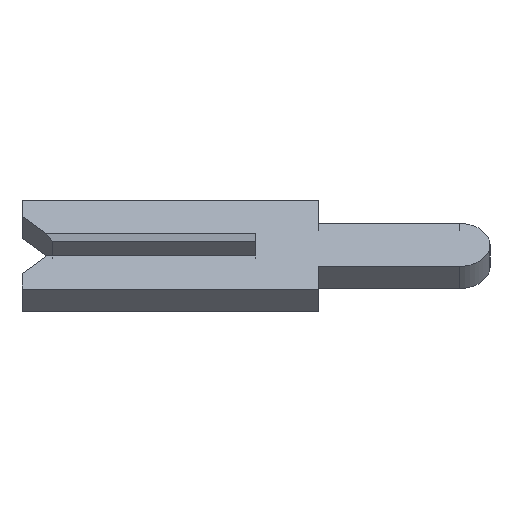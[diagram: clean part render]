
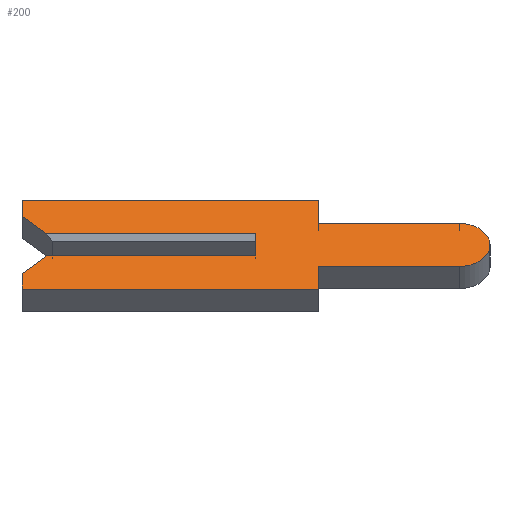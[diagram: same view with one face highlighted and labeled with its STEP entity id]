
A CAD part, left-side view. The second image highlights one B-rep face of the part: STEP entity #200.
In plain terms, the highlighted face is planar.
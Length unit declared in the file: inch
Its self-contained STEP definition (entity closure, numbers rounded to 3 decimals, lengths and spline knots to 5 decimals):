
#16 = LINE ( 'NONE', #425, #167 ) ;
#18 = CARTESIAN_POINT ( 'NONE',  ( -0.01, -0.1305, -0.0195 ) ) ;
#24 = ORIENTED_EDGE ( 'NONE', *, *, #143, .F. ) ;
#27 = PLANE ( 'NONE',  #1065 ) ;
#28 = ORIENTED_EDGE ( 'NONE', *, *, #935, .F. ) ;
#33 = LINE ( 'NONE', #1054, #142 ) ;
#55 = ORIENTED_EDGE ( 'NONE', *, *, #101, .F. ) ;
#59 = VERTEX_POINT ( 'NONE', #343 ) ;
#66 = VERTEX_POINT ( 'NONE', #703 ) ;
#69 = ORIENTED_EDGE ( 'NONE', *, *, #1071, .F. ) ;
#80 = DIRECTION ( 'NONE',  ( 1., 0., 0. ) ) ;
#82 = VECTOR ( 'NONE', #792, 39.37008 ) ;
#91 = VECTOR ( 'NONE', #368, 39.37008 ) ;
#98 = DIRECTION ( 'NONE',  ( 0., 0., -1. ) ) ;
#101 = EDGE_CURVE ( 'NONE', #66, #231, #1145, .T. ) ;
#102 = CARTESIAN_POINT ( 'NONE',  ( -0.01, -0.04, 0.0195 ) ) ;
#120 = CARTESIAN_POINT ( 'NONE',  ( -0.01, -0.04, 0.0195 ) ) ;
#132 = DIRECTION ( 'NONE',  ( 0., 0., -1. ) ) ;
#142 = VECTOR ( 'NONE', #684, 39.37008 ) ;
#143 = EDGE_CURVE ( 'NONE', #290, #892, #457, .T. ) ;
#148 = ORIENTED_EDGE ( 'NONE', *, *, #864, .F. ) ;
#152 = LINE ( 'NONE', #506, #410 ) ;
#167 = VECTOR ( 'NONE', #515, 39.37008 ) ;
#176 = CIRCLE ( 'NONE', #236, 0.0195 ) ;
#181 = VECTOR ( 'NONE', #212, 39.37008 ) ;
#185 = CARTESIAN_POINT ( 'NONE',  ( -0.01, 0.15, -0.04 ) ) ;
#200 = ADVANCED_FACE ( 'NONE', ( #809 ), #27, .F. ) ;
#212 = DIRECTION ( 'NONE',  ( 0., 1., 0. ) ) ;
#226 = DIRECTION ( 'NONE',  ( 0., -1., 0. ) ) ;
#231 = VERTEX_POINT ( 'NONE', #642 ) ;
#233 = VERTEX_POINT ( 'NONE', #823 ) ;
#236 = AXIS2_PLACEMENT_3D ( 'NONE', #546, #456, #98 ) ;
#242 = EDGE_CURVE ( 'NONE', #244, #392, #176, .T. ) ;
#244 = VERTEX_POINT ( 'NONE', #452 ) ;
#254 = CARTESIAN_POINT ( 'NONE',  ( -0.01, 0.15, 0.04 ) ) ;
#261 = EDGE_CURVE ( 'NONE', #1116, #59, #404, .T. ) ;
#270 = VERTEX_POINT ( 'NONE', #254 ) ;
#290 = VERTEX_POINT ( 'NONE', #185 ) ;
#294 = VECTOR ( 'NONE', #440, 39.37008 ) ;
#339 = CARTESIAN_POINT ( 'NONE',  ( -0.01, 0.134, 0.01 ) ) ;
#343 = CARTESIAN_POINT ( 'NONE',  ( -0.01, 0., 0.01 ) ) ;
#347 = VERTEX_POINT ( 'NONE', #120 ) ;
#366 = CARTESIAN_POINT ( 'NONE',  ( -0.01, -0.04, -0.04 ) ) ;
#368 = DIRECTION ( 'NONE',  ( 0., -0.707, 0.707 ) ) ;
#380 = VECTOR ( 'NONE', #226, 39.37008 ) ;
#392 = VERTEX_POINT ( 'NONE', #18 ) ;
#404 = LINE ( 'NONE', #1105, #610 ) ;
#410 = VECTOR ( 'NONE', #606, 39.37008 ) ;
#425 = CARTESIAN_POINT ( 'NONE',  ( -0.01, 0.15, 0.04 ) ) ;
#440 = DIRECTION ( 'NONE',  ( 0., 1., 0. ) ) ;
#444 = ORIENTED_EDGE ( 'NONE', *, *, #261, .T. ) ;
#452 = CARTESIAN_POINT ( 'NONE',  ( -0.01, -0.1305, 0.0195 ) ) ;
#456 = DIRECTION ( 'NONE',  ( 1., 0., 0. ) ) ;
#457 = LINE ( 'NONE', #830, #1111 ) ;
#486 = CARTESIAN_POINT ( 'NONE',  ( -0.01, -0.04, -0.0195 ) ) ;
#502 = EDGE_CURVE ( 'NONE', #347, #244, #1008, .T. ) ;
#506 = CARTESIAN_POINT ( 'NONE',  ( -0.01, 0.15, 0.026 ) ) ;
#515 = DIRECTION ( 'NONE',  ( 0., -1., 0. ) ) ;
#524 = CARTESIAN_POINT ( 'NONE',  ( -0.01, 0.15, -0.04 ) ) ;
#546 = CARTESIAN_POINT ( 'NONE',  ( -0.01, -0.1305, 0. ) ) ;
#553 = EDGE_CURVE ( 'NONE', #892, #233, #562, .T. ) ;
#562 = LINE ( 'NONE', #766, #91 ) ;
#588 = EDGE_CURVE ( 'NONE', #233, #1149, #1025, .T. ) ;
#603 = VECTOR ( 'NONE', #132, 39.37008 ) ;
#606 = DIRECTION ( 'NONE',  ( 0., 0., 1. ) ) ;
#607 = EDGE_CURVE ( 'NONE', #392, #66, #846, .T. ) ;
#610 = VECTOR ( 'NONE', #1024, 39.37008 ) ;
#611 = ORIENTED_EDGE ( 'NONE', *, *, #973, .F. ) ;
#628 = VERTEX_POINT ( 'NONE', #981 ) ;
#642 = CARTESIAN_POINT ( 'NONE',  ( -0.01, -0.04, -0.04 ) ) ;
#650 = CARTESIAN_POINT ( 'NONE',  ( -0.01, -0.1305, 0. ) ) ;
#655 = ORIENTED_EDGE ( 'NONE', *, *, #588, .F. ) ;
#666 = VECTOR ( 'NONE', #738, 39.37008 ) ;
#679 = CARTESIAN_POINT ( 'NONE',  ( -0.01, 0.15, -0.026 ) ) ;
#684 = DIRECTION ( 'NONE',  ( 0., 0.707, 0.707 ) ) ;
#695 = ORIENTED_EDGE ( 'NONE', *, *, #773, .F. ) ;
#698 = CARTESIAN_POINT ( 'NONE',  ( -0.01, 0., 0.0065 ) ) ;
#703 = CARTESIAN_POINT ( 'NONE',  ( -0.01, -0.04, -0.0195 ) ) ;
#726 = DIRECTION ( 'NONE',  ( 0., 0., -1. ) ) ;
#738 = DIRECTION ( 'NONE',  ( 0., 0., -1. ) ) ;
#766 = CARTESIAN_POINT ( 'NONE',  ( -0.01, 0.1305, -0.0065 ) ) ;
#773 = EDGE_CURVE ( 'NONE', #1116, #1136, #33, .T. ) ;
#775 = ORIENTED_EDGE ( 'NONE', *, *, #553, .F. ) ;
#780 = CARTESIAN_POINT ( 'NONE',  ( -0.01, -0.1305, -0.01 ) ) ;
#792 = DIRECTION ( 'NONE',  ( 0., 0., 1. ) ) ;
#801 = CARTESIAN_POINT ( 'NONE',  ( -0.01, 0.15, 0.026 ) ) ;
#809 = FACE_OUTER_BOUND ( 'NONE', #966, .T. ) ;
#816 = LINE ( 'NONE', #524, #294 ) ;
#823 = CARTESIAN_POINT ( 'NONE',  ( -0.01, 0.134, -0.01 ) ) ;
#830 = CARTESIAN_POINT ( 'NONE',  ( -0.01, 0.15, -0.026 ) ) ;
#840 = EDGE_CURVE ( 'NONE', #628, #347, #1165, .T. ) ;
#846 = LINE ( 'NONE', #486, #181 ) ;
#854 = ORIENTED_EDGE ( 'NONE', *, *, #607, .F. ) ;
#864 = EDGE_CURVE ( 'NONE', #1149, #59, #969, .T. ) ;
#892 = VERTEX_POINT ( 'NONE', #679 ) ;
#900 = DIRECTION ( 'NONE',  ( 0., 0., 1. ) ) ;
#935 = EDGE_CURVE ( 'NONE', #1136, #270, #152, .T. ) ;
#943 = ORIENTED_EDGE ( 'NONE', *, *, #502, .F. ) ;
#957 = CARTESIAN_POINT ( 'NONE',  ( -0.01, -0.04, 0.04 ) ) ;
#966 = EDGE_LOOP ( 'NONE', ( #444, #148, #655, #775, #24, #611, #55, #854, #994, #943, #1044, #69, #28, #695 ) ) ;
#969 = LINE ( 'NONE', #698, #82 ) ;
#973 = EDGE_CURVE ( 'NONE', #231, #290, #816, .T. ) ;
#981 = CARTESIAN_POINT ( 'NONE',  ( -0.01, -0.04, 0.04 ) ) ;
#994 = ORIENTED_EDGE ( 'NONE', *, *, #242, .F. ) ;
#1008 = LINE ( 'NONE', #102, #1130 ) ;
#1019 = DIRECTION ( 'NONE',  ( 0., -1., 0. ) ) ;
#1024 = DIRECTION ( 'NONE',  ( 0., -1., 0. ) ) ;
#1025 = LINE ( 'NONE', #780, #380 ) ;
#1044 = ORIENTED_EDGE ( 'NONE', *, *, #840, .F. ) ;
#1054 = CARTESIAN_POINT ( 'NONE',  ( -0.01, 0.1305, 0.0065 ) ) ;
#1065 = AXIS2_PLACEMENT_3D ( 'NONE', #650, #80, #726 ) ;
#1071 = EDGE_CURVE ( 'NONE', #270, #628, #16, .T. ) ;
#1105 = CARTESIAN_POINT ( 'NONE',  ( -0.01, 0.15, 0.01 ) ) ;
#1111 = VECTOR ( 'NONE', #900, 39.37008 ) ;
#1116 = VERTEX_POINT ( 'NONE', #339 ) ;
#1130 = VECTOR ( 'NONE', #1019, 39.37008 ) ;
#1136 = VERTEX_POINT ( 'NONE', #801 ) ;
#1145 = LINE ( 'NONE', #366, #666 ) ;
#1149 = VERTEX_POINT ( 'NONE', #1172 ) ;
#1165 = LINE ( 'NONE', #957, #603 ) ;
#1172 = CARTESIAN_POINT ( 'NONE',  ( -0.01, 0., -0.01 ) ) ;
